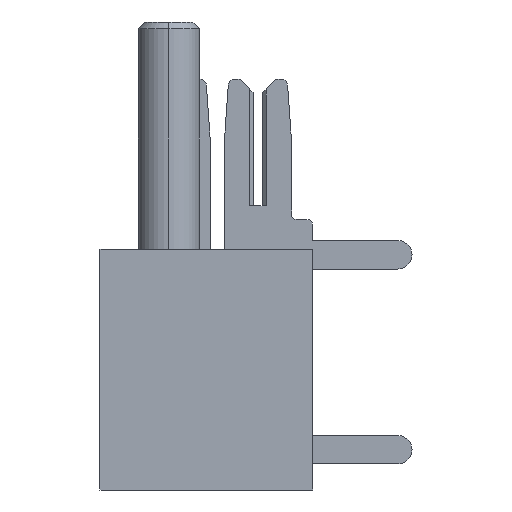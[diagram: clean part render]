
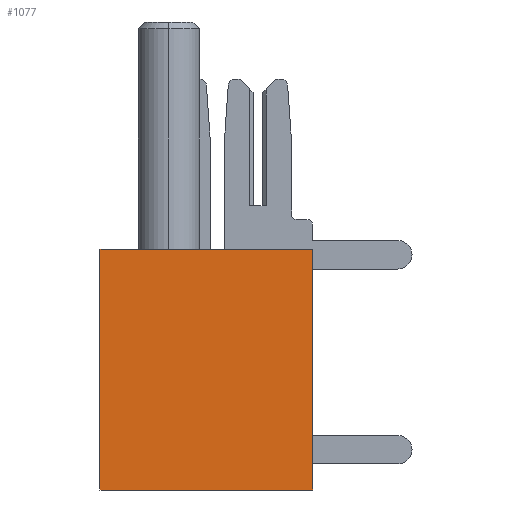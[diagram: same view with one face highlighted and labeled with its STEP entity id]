
A CAD part, left-side view. The second image highlights one B-rep face of the part: STEP entity #1077.
In plain terms, the highlighted planar face has unit normal (-1, 0, 0).
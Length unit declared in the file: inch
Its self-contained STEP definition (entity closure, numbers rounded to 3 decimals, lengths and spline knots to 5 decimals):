
#297 = PLANE ( 'NONE',  #9108 ) ;
#437 = VERTEX_POINT ( 'NONE', #4277 ) ;
#1077 = ADVANCED_FACE ( 'NONE', ( #3722 ), #297, .T. ) ;
#1151 = VECTOR ( 'NONE', #10292, 39.37008 ) ;
#1999 = EDGE_CURVE ( 'NONE', #6305, #437, #10356, .T. ) ;
#2196 = CARTESIAN_POINT ( 'NONE',  ( 0., 0., -0.37 ) ) ;
#2380 = DIRECTION ( 'NONE',  ( 0., 0., 1. ) ) ;
#2978 = CARTESIAN_POINT ( 'NONE',  ( 0., 0.327, -0.37 ) ) ;
#3311 = CARTESIAN_POINT ( 'NONE',  ( 0., 0., -0.37 ) ) ;
#3722 = FACE_OUTER_BOUND ( 'NONE', #4296, .T. ) ;
#4277 = CARTESIAN_POINT ( 'NONE',  ( 0., 0.327, 0. ) ) ;
#4296 = EDGE_LOOP ( 'NONE', ( #8938, #5544, #13263, #13297 ) ) ;
#4423 = LINE ( 'NONE', #7216, #12338 ) ;
#4859 = VERTEX_POINT ( 'NONE', #11291 ) ;
#5544 = ORIENTED_EDGE ( 'NONE', *, *, #1999, .F. ) ;
#5850 = LINE ( 'NONE', #12329, #1151 ) ;
#6166 = VECTOR ( 'NONE', #10829, 39.37008 ) ;
#6305 = VERTEX_POINT ( 'NONE', #10997 ) ;
#6534 = CARTESIAN_POINT ( 'NONE',  ( 0., 0., -0.37 ) ) ;
#6536 = EDGE_CURVE ( 'NONE', #437, #4859, #4423, .T. ) ;
#6951 = VECTOR ( 'NONE', #8197, 39.37008 ) ;
#7142 = EDGE_CURVE ( 'NONE', #9427, #4859, #11366, .T. ) ;
#7216 = CARTESIAN_POINT ( 'NONE',  ( 0., 0., 0. ) ) ;
#8197 = DIRECTION ( 'NONE',  ( 0., 0., 1. ) ) ;
#8253 = DIRECTION ( 'NONE',  ( 0., -1., 0. ) ) ;
#8938 = ORIENTED_EDGE ( 'NONE', *, *, #6536, .F. ) ;
#9108 = AXIS2_PLACEMENT_3D ( 'NONE', #2196, #9508, #2380 ) ;
#9427 = VERTEX_POINT ( 'NONE', #6534 ) ;
#9508 = DIRECTION ( 'NONE',  ( -1., 0., 0. ) ) ;
#10292 = DIRECTION ( 'NONE',  ( 0., -1., 0. ) ) ;
#10356 = LINE ( 'NONE', #2978, #6951 ) ;
#10829 = DIRECTION ( 'NONE',  ( 0., 0., 1. ) ) ;
#10997 = CARTESIAN_POINT ( 'NONE',  ( 0., 0.327, -0.37 ) ) ;
#11291 = CARTESIAN_POINT ( 'NONE',  ( 0., 0., 0. ) ) ;
#11366 = LINE ( 'NONE', #3311, #6166 ) ;
#12329 = CARTESIAN_POINT ( 'NONE',  ( 0., 0., -0.37 ) ) ;
#12338 = VECTOR ( 'NONE', #8253, 39.37008 ) ;
#12903 = EDGE_CURVE ( 'NONE', #6305, #9427, #5850, .T. ) ;
#13263 = ORIENTED_EDGE ( 'NONE', *, *, #12903, .T. ) ;
#13297 = ORIENTED_EDGE ( 'NONE', *, *, #7142, .T. ) ;
